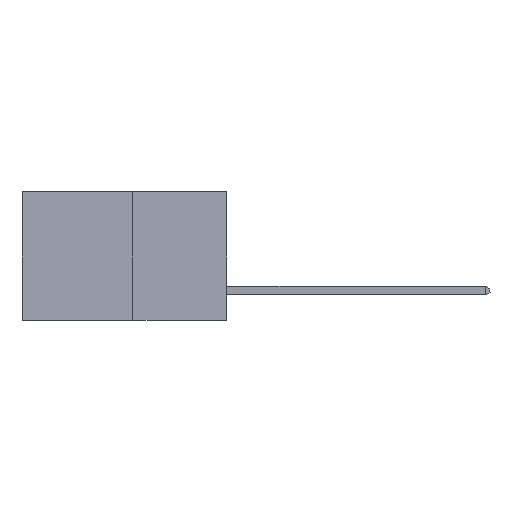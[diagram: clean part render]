
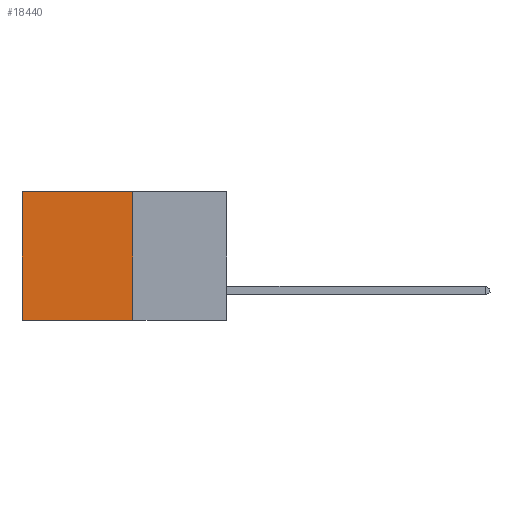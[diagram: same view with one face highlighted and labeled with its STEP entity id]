
A CAD part, left-side view. The second image highlights one B-rep face of the part: STEP entity #18440.
In plain terms, the highlighted planar face has unit normal (-1, 0, 0).
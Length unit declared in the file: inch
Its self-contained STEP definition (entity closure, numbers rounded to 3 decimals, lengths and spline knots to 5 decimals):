
#39 = VERTEX_POINT ( 'NONE', #16265 ) ;
#170 = CARTESIAN_POINT ( 'NONE',  ( 0.277, 0.27, -0.37 ) ) ;
#1480 = DIRECTION ( 'NONE',  ( 0., 1., 0. ) ) ;
#2231 = DIRECTION ( 'NONE',  ( 0., 0., -1. ) ) ;
#2317 = EDGE_CURVE ( 'NONE', #21406, #6001, #19104, .T. ) ;
#2527 = VECTOR ( 'NONE', #2937, 39.37008 ) ;
#2928 = VECTOR ( 'NONE', #1480, 39.37008 ) ;
#2935 = CARTESIAN_POINT ( 'NONE',  ( 0.277, 0.27, 0. ) ) ;
#2937 = DIRECTION ( 'NONE',  ( 0., 0., -1. ) ) ;
#3289 = LINE ( 'NONE', #2935, #24084 ) ;
#3539 = EDGE_LOOP ( 'NONE', ( #7126, #23001, #11737, #8993 ) ) ;
#6001 = VERTEX_POINT ( 'NONE', #17287 ) ;
#6608 = CARTESIAN_POINT ( 'NONE',  ( 0.277, 0.27, -0.37 ) ) ;
#6805 = EDGE_CURVE ( 'NONE', #13862, #6001, #12655, .T. ) ;
#7048 = CARTESIAN_POINT ( 'NONE',  ( 0.277, 0.59, 0. ) ) ;
#7126 = ORIENTED_EDGE ( 'NONE', *, *, #6805, .T. ) ;
#8993 = ORIENTED_EDGE ( 'NONE', *, *, #13125, .T. ) ;
#10338 = AXIS2_PLACEMENT_3D ( 'NONE', #19930, #11870, #25835 ) ;
#11737 = ORIENTED_EDGE ( 'NONE', *, *, #19794, .F. ) ;
#11870 = DIRECTION ( 'NONE',  ( 1., 0., 0. ) ) ;
#12655 = LINE ( 'NONE', #12999, #2527 ) ;
#12999 = CARTESIAN_POINT ( 'NONE',  ( 0.277, 0.59, -0.37 ) ) ;
#13125 = EDGE_CURVE ( 'NONE', #39, #13862, #3289, .T. ) ;
#13753 = LINE ( 'NONE', #170, #23801 ) ;
#13862 = VERTEX_POINT ( 'NONE', #7048 ) ;
#14378 = CARTESIAN_POINT ( 'NONE',  ( 0.277, 0.27, -0.37 ) ) ;
#15073 = DIRECTION ( 'NONE',  ( 0., 1., 0. ) ) ;
#16265 = CARTESIAN_POINT ( 'NONE',  ( 0.277, 0.27, 0. ) ) ;
#17287 = CARTESIAN_POINT ( 'NONE',  ( 0.277, 0.59, -0.37 ) ) ;
#18440 = ADVANCED_FACE ( 'NONE', ( #22287 ), #23872, .F. ) ;
#19104 = LINE ( 'NONE', #14378, #2928 ) ;
#19794 = EDGE_CURVE ( 'NONE', #39, #21406, #13753, .T. ) ;
#19930 = CARTESIAN_POINT ( 'NONE',  ( 0.277, 0.27, -0.37 ) ) ;
#21406 = VERTEX_POINT ( 'NONE', #6608 ) ;
#22287 = FACE_OUTER_BOUND ( 'NONE', #3539, .T. ) ;
#23001 = ORIENTED_EDGE ( 'NONE', *, *, #2317, .F. ) ;
#23801 = VECTOR ( 'NONE', #2231, 39.37008 ) ;
#23872 = PLANE ( 'NONE',  #10338 ) ;
#24084 = VECTOR ( 'NONE', #15073, 39.37008 ) ;
#25835 = DIRECTION ( 'NONE',  ( 0., 0., -1. ) ) ;
